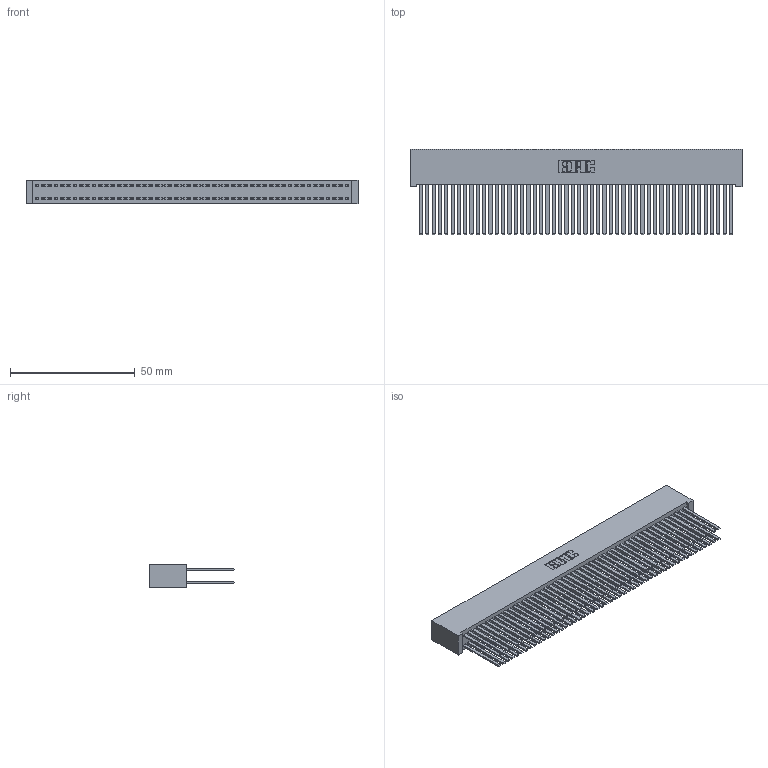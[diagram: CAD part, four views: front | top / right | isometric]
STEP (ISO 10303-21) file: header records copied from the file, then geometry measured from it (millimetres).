
FILE_DESCRIPTION (( 'STEP AP203' ), '1' );
FILE_NAME ('392-100-544-201.STEP', '2018-08-18T18:23:06', ( '' ), ( '' ), 'SwSTEP 2.0', 'SolidWorks 2016', '' );
FILE_SCHEMA (( 'CONFIG_CONTROL_DESIGN' ));
Length unit declared in the file: inch
Products named in the file (3): 345-292-001_345-293-144; 392-100-544-201; 342 Part_Lugless
Assembly tree (101 placements, depth 2):
  392-100-544-201
    342 Part_Lugless
    345-292-001_345-293-144  x100
Bounding box: 133.25 x 34.3 x 9.4 mm (x, y, z)
Volume: 13851.5 mm3; surface area: 27072.3 mm2
Topology: 101 solids, 101 shells, 4702 faces, 13975 edges, 9182 vertices
Faces by surface type: plane 3262, cylinder 1440
Entity records: 30539 total; most frequent: CARTESIAN_POINT 5046, ORIENTED_EDGE 4982, DIRECTION 4287, EDGE_CURVE 2491, LINE 2375, VECTOR 2375, VERTEX_POINT 1658, AXIS2_PLACEMENT_3D 956
